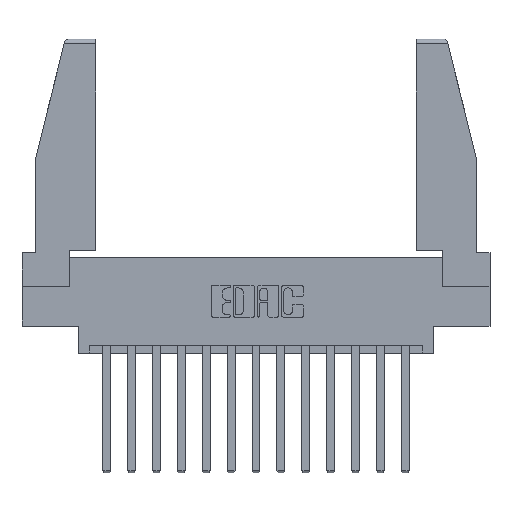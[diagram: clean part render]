
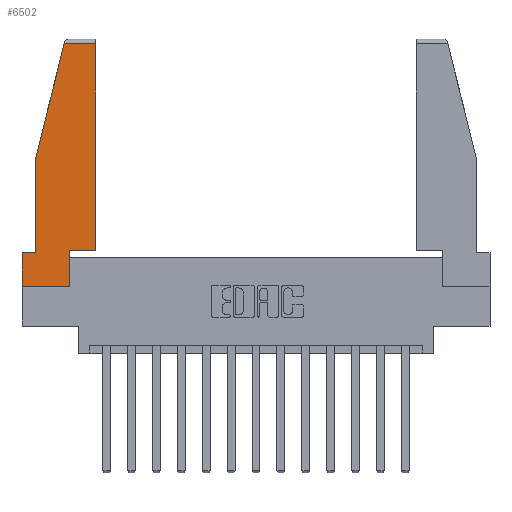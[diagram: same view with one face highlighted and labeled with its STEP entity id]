
A CAD part, top view. The second image highlights one B-rep face of the part: STEP entity #6502.
In plain terms, the highlighted planar face has unit normal (0, 0, 1).
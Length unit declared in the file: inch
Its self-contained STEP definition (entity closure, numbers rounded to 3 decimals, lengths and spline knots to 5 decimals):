
#186 = ORIENTED_EDGE ( 'NONE', *, *, #13852, .T. ) ;
#212 = CARTESIAN_POINT ( 'NONE',  ( 0., 0., 0. ) ) ;
#293 = LINE ( 'NONE', #15775, #13636 ) ;
#411 = CARTESIAN_POINT ( 'NONE',  ( 0.086, 0.8, 0. ) ) ;
#509 = ORIENTED_EDGE ( 'NONE', *, *, #2385, .T. ) ;
#698 = DIRECTION ( 'NONE',  ( 0., -1., 0. ) ) ;
#894 = LINE ( 'NONE', #8943, #8739 ) ;
#1149 = CARTESIAN_POINT ( 'NONE',  ( 0.297, 0., 0. ) ) ;
#1306 = VERTEX_POINT ( 'NONE', #5764 ) ;
#1492 = CARTESIAN_POINT ( 'NONE',  ( 0., 0., 0. ) ) ;
#1744 = DIRECTION ( 'NONE',  ( -1., 0., 0. ) ) ;
#2385 = EDGE_CURVE ( 'NONE', #8093, #3017, #11621, .T. ) ;
#2469 = DIRECTION ( 'NONE',  ( 0., 0., 1. ) ) ;
#3017 = VERTEX_POINT ( 'NONE', #7069 ) ;
#3230 = DIRECTION ( 'NONE',  ( 1., 0., 0. ) ) ;
#3372 = DIRECTION ( 'NONE',  ( 0., 1., 0. ) ) ;
#3427 = LINE ( 'NONE', #9088, #15551 ) ;
#3577 = CARTESIAN_POINT ( 'NONE',  ( 0.086, 0.21, 0. ) ) ;
#3660 = EDGE_CURVE ( 'NONE', #13963, #8299, #3781, .T. ) ;
#3781 = LINE ( 'NONE', #5413, #4971 ) ;
#4509 = CARTESIAN_POINT ( 'NONE',  ( 0., 0.21, 0. ) ) ;
#4523 = VERTEX_POINT ( 'NONE', #13294 ) ;
#4651 = EDGE_CURVE ( 'NONE', #4523, #10401, #894, .T. ) ;
#4971 = VECTOR ( 'NONE', #7894, 39.37008 ) ;
#5102 = EDGE_CURVE ( 'NONE', #10401, #13963, #293, .T. ) ;
#5113 = DIRECTION ( 'NONE',  ( -0.239, -0.971, 0. ) ) ;
#5186 = FACE_OUTER_BOUND ( 'NONE', #9926, .T. ) ;
#5413 = CARTESIAN_POINT ( 'NONE',  ( 0., 0.21, 0. ) ) ;
#5764 = CARTESIAN_POINT ( 'NONE',  ( 0.461, 1.52, 0. ) ) ;
#6502 = ADVANCED_FACE ( 'NONE', ( #5186 ), #8654, .T. ) ;
#6891 = CARTESIAN_POINT ( 'NONE',  ( 0., 0.21, 0. ) ) ;
#7069 = CARTESIAN_POINT ( 'NONE',  ( 0.461, 0.223, 0. ) ) ;
#7151 = DIRECTION ( 'NONE',  ( 0., -1., 0. ) ) ;
#7499 = LINE ( 'NONE', #9563, #14967 ) ;
#7656 = DIRECTION ( 'NONE',  ( 1., 0., 0. ) ) ;
#7826 = DIRECTION ( 'NONE',  ( 1., 0., 0. ) ) ;
#7894 = DIRECTION ( 'NONE',  ( -1., 0., 0. ) ) ;
#8093 = VERTEX_POINT ( 'NONE', #9303 ) ;
#8299 = VERTEX_POINT ( 'NONE', #4509 ) ;
#8654 = PLANE ( 'NONE',  #13668 ) ;
#8739 = VECTOR ( 'NONE', #5113, 39.37008 ) ;
#8943 = CARTESIAN_POINT ( 'NONE',  ( 0.271, 1.55, 0. ) ) ;
#9082 = VERTEX_POINT ( 'NONE', #1492 ) ;
#9088 = CARTESIAN_POINT ( 'NONE',  ( 0., 1.52, 0. ) ) ;
#9303 = CARTESIAN_POINT ( 'NONE',  ( 0.297, 0.223, 0. ) ) ;
#9367 = VECTOR ( 'NONE', #9647, 39.37008 ) ;
#9563 = CARTESIAN_POINT ( 'NONE',  ( 0.297, 0., 0. ) ) ;
#9569 = ORIENTED_EDGE ( 'NONE', *, *, #14470, .T. ) ;
#9647 = DIRECTION ( 'NONE',  ( 0., 1., 0. ) ) ;
#9926 = EDGE_LOOP ( 'NONE', ( #10872, #13546, #13030, #12353, #11439, #186, #12033, #9569, #509 ) ) ;
#10296 = EDGE_CURVE ( 'NONE', #1306, #4523, #3427, .T. ) ;
#10401 = VERTEX_POINT ( 'NONE', #411 ) ;
#10489 = VERTEX_POINT ( 'NONE', #1149 ) ;
#10660 = LINE ( 'NONE', #212, #13603 ) ;
#10872 = ORIENTED_EDGE ( 'NONE', *, *, #12644, .T. ) ;
#11184 = CARTESIAN_POINT ( 'NONE',  ( 0., 0., 0. ) ) ;
#11439 = ORIENTED_EDGE ( 'NONE', *, *, #3660, .T. ) ;
#11463 = VECTOR ( 'NONE', #698, 39.37008 ) ;
#11621 = LINE ( 'NONE', #15655, #14133 ) ;
#12032 = LINE ( 'NONE', #6891, #11463 ) ;
#12033 = ORIENTED_EDGE ( 'NONE', *, *, #14291, .T. ) ;
#12169 = CARTESIAN_POINT ( 'NONE',  ( 0.461, 0.223, 0. ) ) ;
#12353 = ORIENTED_EDGE ( 'NONE', *, *, #5102, .T. ) ;
#12644 = EDGE_CURVE ( 'NONE', #3017, #1306, #15064, .T. ) ;
#13030 = ORIENTED_EDGE ( 'NONE', *, *, #4651, .T. ) ;
#13294 = CARTESIAN_POINT ( 'NONE',  ( 0.2636, 1.52, 0. ) ) ;
#13546 = ORIENTED_EDGE ( 'NONE', *, *, #10296, .T. ) ;
#13603 = VECTOR ( 'NONE', #7826, 39.37008 ) ;
#13636 = VECTOR ( 'NONE', #7151, 39.37008 ) ;
#13668 = AXIS2_PLACEMENT_3D ( 'NONE', #11184, #2469, #7656 ) ;
#13852 = EDGE_CURVE ( 'NONE', #8299, #9082, #12032, .T. ) ;
#13963 = VERTEX_POINT ( 'NONE', #3577 ) ;
#14133 = VECTOR ( 'NONE', #3230, 39.37008 ) ;
#14291 = EDGE_CURVE ( 'NONE', #9082, #10489, #10660, .T. ) ;
#14470 = EDGE_CURVE ( 'NONE', #10489, #8093, #7499, .T. ) ;
#14967 = VECTOR ( 'NONE', #3372, 39.37008 ) ;
#15064 = LINE ( 'NONE', #12169, #9367 ) ;
#15551 = VECTOR ( 'NONE', #1744, 39.37008 ) ;
#15655 = CARTESIAN_POINT ( 'NONE',  ( 0.297, 0.223, 0. ) ) ;
#15775 = CARTESIAN_POINT ( 'NONE',  ( 0.086, 0.8, 0. ) ) ;
